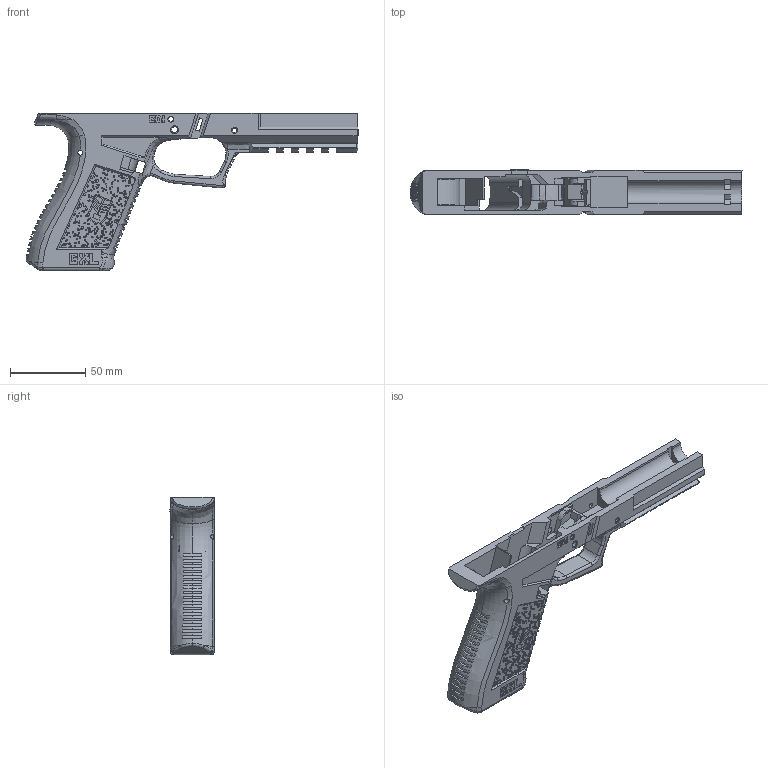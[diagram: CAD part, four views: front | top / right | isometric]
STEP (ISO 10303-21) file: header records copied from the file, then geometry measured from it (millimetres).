
FILE_DESCRIPTION(/* description */ (''),/* implementation_level */ '2;1');
FILE_NAME(/* name */ 'DD17.2 CRUSHER34 Railed.step',/* time_stamp */ '2022-08-30T18:44:18-05:00',/* author */ (''),/* organization */ (''),/* preprocessor_version */ 'ST-DEVELOPER v19',/* originating_system */ 'Autodesk Translation Framework v11.7.0.108',/* authorisation */ '');
FILE_SCHEMA (('AUTOMOTIVE_DESIGN { 1 0 10303 214 3 1 1 }'));
Products named in the file (1): DD17.2 SDI GXL CRUSHER
Bounding box: 220.66 x 29.73 x 104.95 mm (x, y, z)
Volume: 124365.9 mm3; surface area: 56608.6 mm2
Topology: 1 solids, 2 shells, 3446 faces, 9036 edges, 5974 vertices
Faces by surface type: bspline 2287, plane 1083, cylinder 65, torus 11
Full cylindrical faces by diameter (mm): 1.933 x1, 3 x4, 3.2 x2, 3.5 x1, 4.1 x2, 4.5 x2
Entity records: 138554 total; most frequent: CARTESIAN_POINT 75967, ORIENTED_EDGE 18054, EDGE_CURVE 9027, DIRECTION 6585, VERTEX_POINT 5974, EDGE_LOOP 3869, LINE 3763, VECTOR 3763
